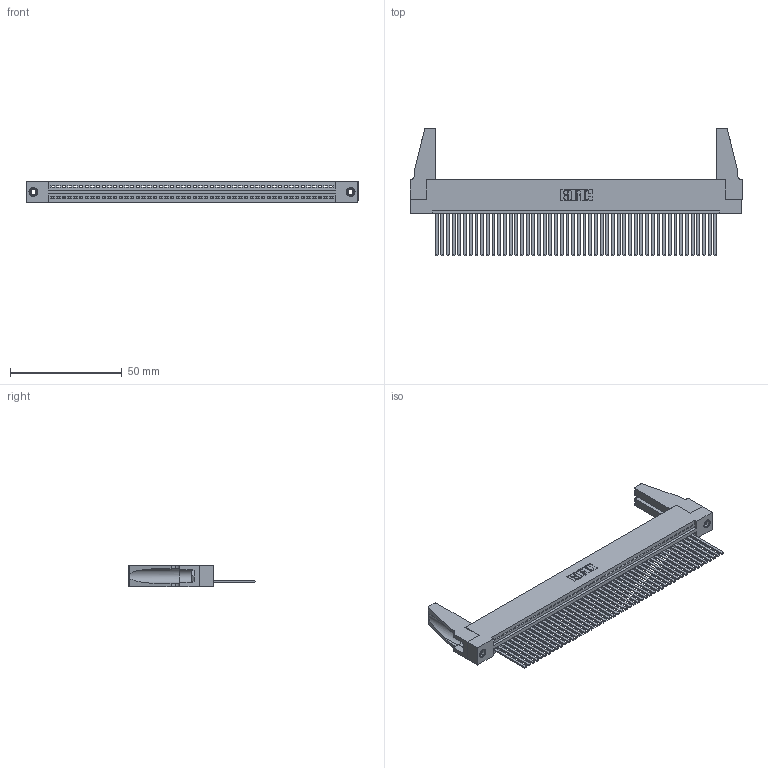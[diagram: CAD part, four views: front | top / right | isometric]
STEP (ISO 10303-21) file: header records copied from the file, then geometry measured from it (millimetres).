
FILE_DESCRIPTION (( 'STEP AP203' ), '1' );
FILE_NAME ('345-050-544-188.STEP', '2019-10-09T13:11:10', ( '' ), ( '' ), 'SwSTEP 2.0', 'SolidWorks 2016', '' );
FILE_SCHEMA (( 'CONFIG_CONTROL_DESIGN' ));
Length unit declared in the file: inch
Products named in the file (5): 345 Part_Flush Mounting Lugs - 0.156 Dia-TH; 345-050-544-188; 345-220-078_345-220-088; 345-292-001_345-293-144; 345-250-001_345-250-001-102
Assembly tree (55 placements, depth 2):
  345-050-544-188
    345 Part_Flush Mounting Lugs - 0.156 Dia-TH
    345-292-001_345-293-144  x50
    345-250-001_345-250-001-102  x2
    345-220-078_345-220-088  x2
Bounding box: 148.23 x 56.82 x 9.4 mm (x, y, z)
Volume: 17976.5 mm3; surface area: 24543.3 mm2
Topology: 55 solids, 55 shells, 2850 faces, 8555 edges, 5626 vertices
Faces by surface type: plane 1952, cylinder 882, cone 12, torus 4
Entity records: 38518 total; most frequent: CARTESIAN_POINT 6660, ORIENTED_EDGE 6604, DIRECTION 5810, EDGE_CURVE 3302, VECTOR 2932, LINE 2932, VERTEX_POINT 2194, AXIS2_PLACEMENT_3D 1439
